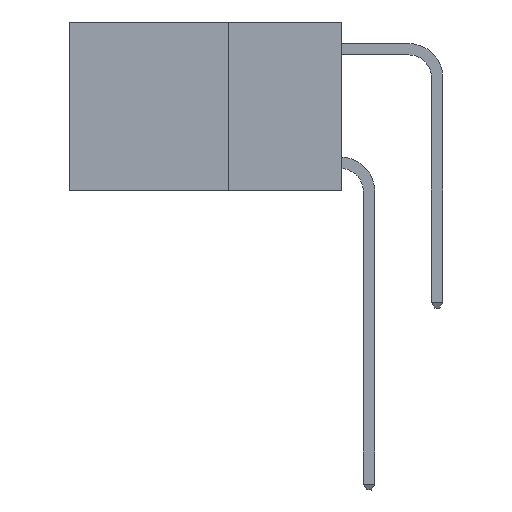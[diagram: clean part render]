
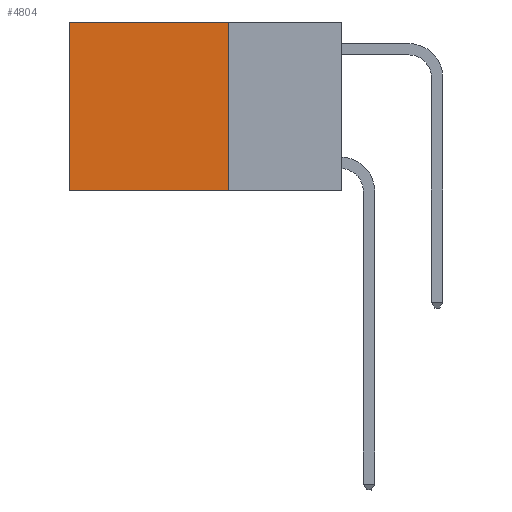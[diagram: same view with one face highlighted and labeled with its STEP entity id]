
A CAD part, left-side view. The second image highlights one B-rep face of the part: STEP entity #4804.
In plain terms, the highlighted planar face has unit normal (-1, 0, 0).
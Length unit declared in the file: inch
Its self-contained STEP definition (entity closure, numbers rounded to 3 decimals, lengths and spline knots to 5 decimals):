
#69 = CARTESIAN_POINT ( 'NONE',  ( 0.2625, 0.25, 0. ) ) ;
#148 = VERTEX_POINT ( 'NONE', #4105 ) ;
#536 = ORIENTED_EDGE ( 'NONE', *, *, #5030, .T. ) ;
#1724 = DIRECTION ( 'NONE',  ( 0., 1., 0. ) ) ;
#1944 = LINE ( 'NONE', #9952, #9470 ) ;
#2002 = VECTOR ( 'NONE', #1724, 39.37008 ) ;
#2196 = EDGE_LOOP ( 'NONE', ( #7154, #10513, #5205, #536 ) ) ;
#2332 = LINE ( 'NONE', #7919, #2002 ) ;
#3302 = LINE ( 'NONE', #9730, #8364 ) ;
#3557 = CARTESIAN_POINT ( 'NONE',  ( 0.2625, 0.25, 0. ) ) ;
#3840 = VERTEX_POINT ( 'NONE', #8241 ) ;
#4105 = CARTESIAN_POINT ( 'NONE',  ( 0.2625, 0.6, 0. ) ) ;
#4577 = CARTESIAN_POINT ( 'NONE',  ( 0.2625, 0.25, 0. ) ) ;
#4804 = ADVANCED_FACE ( 'NONE', ( #7032 ), #6548, .F. ) ;
#5030 = EDGE_CURVE ( 'NONE', #8619, #148, #2332, .T. ) ;
#5205 = ORIENTED_EDGE ( 'NONE', *, *, #6340, .F. ) ;
#5582 = DIRECTION ( 'NONE',  ( 0., 0., -1. ) ) ;
#5702 = AXIS2_PLACEMENT_3D ( 'NONE', #4577, #11648, #5582 ) ;
#6340 = EDGE_CURVE ( 'NONE', #8619, #7419, #10147, .T. ) ;
#6548 = PLANE ( 'NONE',  #5702 ) ;
#6858 = EDGE_CURVE ( 'NONE', #7419, #3840, #3302, .T. ) ;
#7032 = FACE_OUTER_BOUND ( 'NONE', #2196, .T. ) ;
#7141 = VECTOR ( 'NONE', #8505, 39.37008 ) ;
#7154 = ORIENTED_EDGE ( 'NONE', *, *, #12889, .T. ) ;
#7419 = VERTEX_POINT ( 'NONE', #10660 ) ;
#7919 = CARTESIAN_POINT ( 'NONE',  ( 0.2625, 0.25, 0. ) ) ;
#8241 = CARTESIAN_POINT ( 'NONE',  ( 0.2625, 0.6, -0.37 ) ) ;
#8364 = VECTOR ( 'NONE', #10770, 39.37008 ) ;
#8505 = DIRECTION ( 'NONE',  ( 0., 0., -1. ) ) ;
#8619 = VERTEX_POINT ( 'NONE', #3557 ) ;
#9470 = VECTOR ( 'NONE', #12922, 39.37008 ) ;
#9730 = CARTESIAN_POINT ( 'NONE',  ( 0.2625, 0.25, -0.37 ) ) ;
#9952 = CARTESIAN_POINT ( 'NONE',  ( 0.2625, 0.6, 0. ) ) ;
#10147 = LINE ( 'NONE', #69, #7141 ) ;
#10513 = ORIENTED_EDGE ( 'NONE', *, *, #6858, .F. ) ;
#10660 = CARTESIAN_POINT ( 'NONE',  ( 0.2625, 0.25, -0.37 ) ) ;
#10770 = DIRECTION ( 'NONE',  ( 0., 1., 0. ) ) ;
#11648 = DIRECTION ( 'NONE',  ( 1., 0., 0. ) ) ;
#12889 = EDGE_CURVE ( 'NONE', #148, #3840, #1944, .T. ) ;
#12922 = DIRECTION ( 'NONE',  ( 0., 0., -1. ) ) ;
